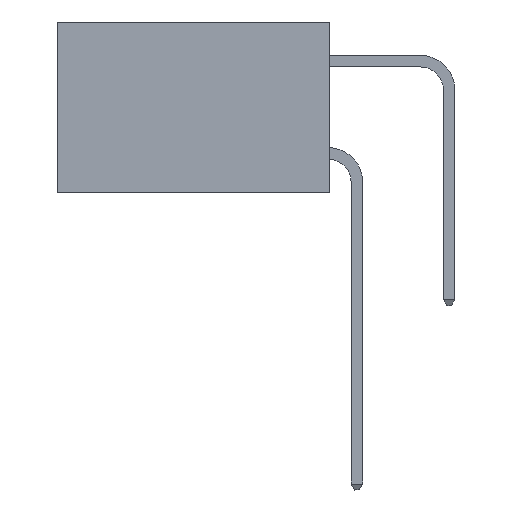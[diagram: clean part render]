
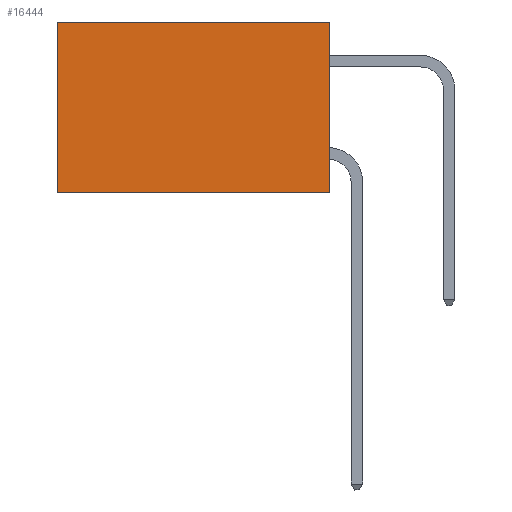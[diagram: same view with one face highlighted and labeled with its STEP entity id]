
A CAD part, left-side view. The second image highlights one B-rep face of the part: STEP entity #16444.
In plain terms, the highlighted planar face has unit normal (-1, 0, 0).
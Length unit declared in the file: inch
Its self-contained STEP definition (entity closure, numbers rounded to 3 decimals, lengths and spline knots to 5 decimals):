
#702 = CARTESIAN_POINT ( 'NONE',  ( 0.277, 0.59, -0.37 ) ) ;
#1882 = CARTESIAN_POINT ( 'NONE',  ( 0.277, 0., 0. ) ) ;
#1962 = VECTOR ( 'NONE', #11786, 39.37008 ) ;
#3018 = ORIENTED_EDGE ( 'NONE', *, *, #14379, .T. ) ;
#3095 = CARTESIAN_POINT ( 'NONE',  ( 0.277, 0., -0.37 ) ) ;
#3223 = VECTOR ( 'NONE', #15297, 39.37008 ) ;
#4196 = EDGE_LOOP ( 'NONE', ( #13696, #13661, #5234, #3018 ) ) ;
#4955 = DIRECTION ( 'NONE',  ( 0., 1., 0. ) ) ;
#5234 = ORIENTED_EDGE ( 'NONE', *, *, #19328, .F. ) ;
#5327 = CARTESIAN_POINT ( 'NONE',  ( 0.277, 0.59, -0.37 ) ) ;
#5904 = VERTEX_POINT ( 'NONE', #1882 ) ;
#6356 = CARTESIAN_POINT ( 'NONE',  ( 0.277, 0., 0. ) ) ;
#7128 = CARTESIAN_POINT ( 'NONE',  ( 0.277, 0., -0.37 ) ) ;
#9954 = FACE_OUTER_BOUND ( 'NONE', #4196, .T. ) ;
#10610 = VERTEX_POINT ( 'NONE', #5327 ) ;
#11670 = VECTOR ( 'NONE', #4955, 39.37008 ) ;
#11786 = DIRECTION ( 'NONE',  ( 0., 1., 0. ) ) ;
#11791 = DIRECTION ( 'NONE',  ( 0., 0., -1. ) ) ;
#12270 = LINE ( 'NONE', #6356, #1962 ) ;
#13498 = PLANE ( 'NONE',  #14382 ) ;
#13661 = ORIENTED_EDGE ( 'NONE', *, *, #22769, .F. ) ;
#13696 = ORIENTED_EDGE ( 'NONE', *, *, #13904, .T. ) ;
#13904 = EDGE_CURVE ( 'NONE', #22785, #10610, #16420, .T. ) ;
#14379 = EDGE_CURVE ( 'NONE', #5904, #22785, #12270, .T. ) ;
#14382 = AXIS2_PLACEMENT_3D ( 'NONE', #20557, #22279, #11791 ) ;
#15297 = DIRECTION ( 'NONE',  ( 0., 0., -1. ) ) ;
#16072 = DIRECTION ( 'NONE',  ( 0., 0., -1. ) ) ;
#16261 = VERTEX_POINT ( 'NONE', #20130 ) ;
#16420 = LINE ( 'NONE', #702, #3223 ) ;
#16444 = ADVANCED_FACE ( 'NONE', ( #9954 ), #13498, .F. ) ;
#16516 = VECTOR ( 'NONE', #16072, 39.37008 ) ;
#17084 = LINE ( 'NONE', #7128, #16516 ) ;
#19258 = CARTESIAN_POINT ( 'NONE',  ( 0.277, 0.59, 0. ) ) ;
#19328 = EDGE_CURVE ( 'NONE', #5904, #16261, #17084, .T. ) ;
#20130 = CARTESIAN_POINT ( 'NONE',  ( 0.277, 0., -0.37 ) ) ;
#20557 = CARTESIAN_POINT ( 'NONE',  ( 0.277, 0., -0.37 ) ) ;
#21004 = LINE ( 'NONE', #3095, #11670 ) ;
#22279 = DIRECTION ( 'NONE',  ( 1., 0., 0. ) ) ;
#22769 = EDGE_CURVE ( 'NONE', #16261, #10610, #21004, .T. ) ;
#22785 = VERTEX_POINT ( 'NONE', #19258 ) ;
